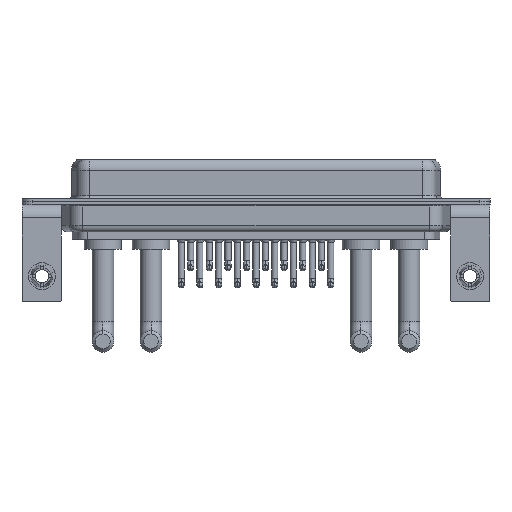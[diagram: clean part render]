
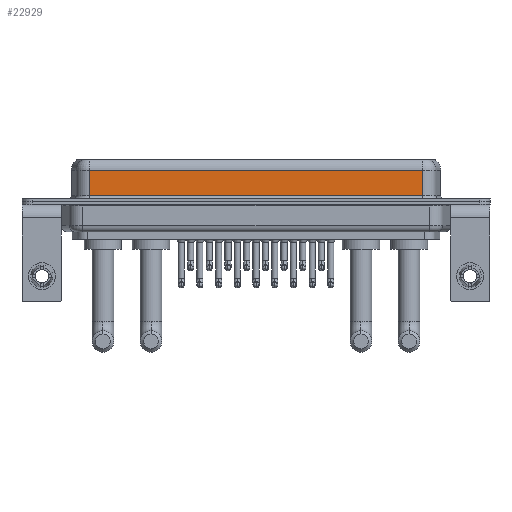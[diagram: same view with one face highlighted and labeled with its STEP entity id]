
A CAD part, front view. The second image highlights one B-rep face of the part: STEP entity #22929.
In plain terms, the highlighted planar face has unit normal (0, -1, 0).
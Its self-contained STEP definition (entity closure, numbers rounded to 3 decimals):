
#551 = ORIENTED_EDGE ( 'NONE', *, *, #20046, .F. ) ;
#1029 = AXIS2_PLACEMENT_3D ( 'NONE', #14520, #7094, #20445 ) ;
#1183 = VERTEX_POINT ( 'NONE', #11248 ) ;
#2060 = VERTEX_POINT ( 'NONE', #7365 ) ;
#2097 = ORIENTED_EDGE ( 'NONE', *, *, #12947, .T. ) ;
#2880 = EDGE_CURVE ( 'NONE', #17705, #2060, #4055, .T. ) ;
#3282 = VECTOR ( 'NONE', #16709, 1000. ) ;
#3487 = LINE ( 'NONE', #14854, #3282 ) ;
#3774 = VERTEX_POINT ( 'NONE', #23896 ) ;
#4055 = LINE ( 'NONE', #17037, #11322 ) ;
#5439 = VECTOR ( 'NONE', #19038, 1000. ) ;
#5714 = ORIENTED_EDGE ( 'NONE', *, *, #2880, .T. ) ;
#6153 = DIRECTION ( 'NONE',  ( 1., 0., 0. ) ) ;
#6533 = EDGE_CURVE ( 'NONE', #1183, #3774, #16245, .T. ) ;
#7094 = DIRECTION ( 'NONE',  ( 0., 1., 0. ) ) ;
#7365 = CARTESIAN_POINT ( 'NONE',  ( 56.462, -3.95, 0.9 ) ) ;
#11248 = CARTESIAN_POINT ( 'NONE',  ( 56.462, -3.95, 4.65 ) ) ;
#11322 = VECTOR ( 'NONE', #6153, 1000. ) ;
#11627 = LINE ( 'NONE', #13722, #5439 ) ;
#12773 = DIRECTION ( 'NONE',  ( -1., 0., 0. ) ) ;
#12947 = EDGE_CURVE ( 'NONE', #3774, #17705, #11627, .T. ) ;
#13722 = CARTESIAN_POINT ( 'NONE',  ( 7.038, -3.95, 6.4 ) ) ;
#14171 = EDGE_LOOP ( 'NONE', ( #551, #14734, #2097, #5714 ) ) ;
#14520 = CARTESIAN_POINT ( 'NONE',  ( 56.462, -3.95, 6.4 ) ) ;
#14734 = ORIENTED_EDGE ( 'NONE', *, *, #6533, .T. ) ;
#14854 = CARTESIAN_POINT ( 'NONE',  ( 56.462, -3.95, 6.4 ) ) ;
#15634 = CARTESIAN_POINT ( 'NONE',  ( 7.038, -3.95, 0.9 ) ) ;
#16245 = LINE ( 'NONE', #22042, #23646 ) ;
#16709 = DIRECTION ( 'NONE',  ( 0., 0., -1. ) ) ;
#17037 = CARTESIAN_POINT ( 'NONE',  ( 56.462, -3.95, 0.9 ) ) ;
#17705 = VERTEX_POINT ( 'NONE', #15634 ) ;
#19038 = DIRECTION ( 'NONE',  ( 0., 0., -1. ) ) ;
#20046 = EDGE_CURVE ( 'NONE', #1183, #2060, #3487, .T. ) ;
#20445 = DIRECTION ( 'NONE',  ( 0., 0., 1. ) ) ;
#22042 = CARTESIAN_POINT ( 'NONE',  ( 56.462, -3.95, 4.65 ) ) ;
#22052 = FACE_OUTER_BOUND ( 'NONE', #14171, .T. ) ;
#22174 = PLANE ( 'NONE',  #1029 ) ;
#22929 = ADVANCED_FACE ( 'NONE', ( #22052 ), #22174, .F. ) ;
#23646 = VECTOR ( 'NONE', #12773, 1000. ) ;
#23896 = CARTESIAN_POINT ( 'NONE',  ( 7.038, -3.95, 4.65 ) ) ;
